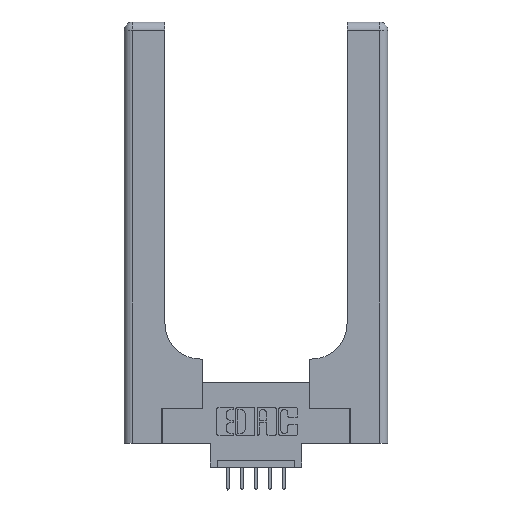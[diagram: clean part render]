
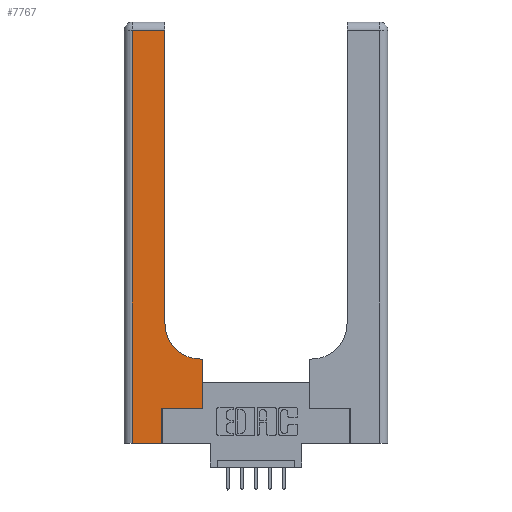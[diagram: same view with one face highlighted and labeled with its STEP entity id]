
A CAD part, top view. The second image highlights one B-rep face of the part: STEP entity #7767.
In plain terms, the highlighted planar face has unit normal (0, 0, 1).
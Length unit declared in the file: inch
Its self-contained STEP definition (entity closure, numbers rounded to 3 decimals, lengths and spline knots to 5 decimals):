
#170 = CARTESIAN_POINT ( 'NONE',  ( 0.5585, 0.6, 0.37 ) ) ;
#234 = DIRECTION ( 'NONE',  ( 0., 1., 0. ) ) ;
#961 = DIRECTION ( 'NONE',  ( 0., -1., 0. ) ) ;
#978 = DIRECTION ( 'NONE',  ( 0., 1., 0. ) ) ;
#1142 = LINE ( 'NONE', #6953, #4225 ) ;
#1166 = VECTOR ( 'NONE', #961, 39.37008 ) ;
#1433 = CIRCLE ( 'NONE', #10699, 0.25 ) ;
#1473 = LINE ( 'NONE', #1996, #12757 ) ;
#1967 = EDGE_CURVE ( 'NONE', #4353, #11476, #1142, .T. ) ;
#1996 = CARTESIAN_POINT ( 'NONE',  ( 0.269, 0.25, 0.37 ) ) ;
#2134 = ORIENTED_EDGE ( 'NONE', *, *, #12451, .T. ) ;
#2267 = PLANE ( 'NONE',  #4599 ) ;
#2344 = ORIENTED_EDGE ( 'NONE', *, *, #4306, .T. ) ;
#2591 = ORIENTED_EDGE ( 'NONE', *, *, #8455, .T. ) ;
#2785 = ORIENTED_EDGE ( 'NONE', *, *, #5712, .T. ) ;
#2977 = VERTEX_POINT ( 'NONE', #9577 ) ;
#3075 = CARTESIAN_POINT ( 'NONE',  ( 0.06, 3., 0.37 ) ) ;
#3300 = LINE ( 'NONE', #5132, #11838 ) ;
#3360 = CARTESIAN_POINT ( 'NONE',  ( 0., 3., 0.37 ) ) ;
#3619 = CARTESIAN_POINT ( 'NONE',  ( 0.2915, 2.94, 0.37 ) ) ;
#3809 = CARTESIAN_POINT ( 'NONE',  ( 0., 2.94, 0.37 ) ) ;
#3987 = EDGE_CURVE ( 'NONE', #8454, #4376, #9463, .T. ) ;
#4225 = VECTOR ( 'NONE', #6894, 39.37008 ) ;
#4274 = VERTEX_POINT ( 'NONE', #13783 ) ;
#4306 = EDGE_CURVE ( 'NONE', #11476, #5413, #4666, .T. ) ;
#4353 = VERTEX_POINT ( 'NONE', #14012 ) ;
#4376 = VERTEX_POINT ( 'NONE', #170 ) ;
#4588 = CARTESIAN_POINT ( 'NONE',  ( 0.2915, 0.6, 0.37 ) ) ;
#4599 = AXIS2_PLACEMENT_3D ( 'NONE', #3360, #6526, #10893 ) ;
#4666 = LINE ( 'NONE', #7544, #11666 ) ;
#4766 = EDGE_CURVE ( 'NONE', #4274, #4353, #7361, .T. ) ;
#5132 = CARTESIAN_POINT ( 'NONE',  ( 0.2915, 3., 0.37 ) ) ;
#5268 = LINE ( 'NONE', #3809, #12948 ) ;
#5413 = VERTEX_POINT ( 'NONE', #13988 ) ;
#5712 = EDGE_CURVE ( 'NONE', #11669, #4274, #5268, .T. ) ;
#5795 = DIRECTION ( 'NONE',  ( -1., 0., 0. ) ) ;
#6062 = VECTOR ( 'NONE', #5795, 39.37008 ) ;
#6109 = DIRECTION ( 'NONE',  ( -1., 0., 0. ) ) ;
#6526 = DIRECTION ( 'NONE',  ( 0., 0., -1. ) ) ;
#6568 = VECTOR ( 'NONE', #234, 39.37008 ) ;
#6671 = ORIENTED_EDGE ( 'NONE', *, *, #3987, .T. ) ;
#6894 = DIRECTION ( 'NONE',  ( 1., 0., 0. ) ) ;
#6953 = CARTESIAN_POINT ( 'NONE',  ( 0., 0., 0.37 ) ) ;
#7361 = LINE ( 'NONE', #3075, #1166 ) ;
#7544 = CARTESIAN_POINT ( 'NONE',  ( 0.269, 0., 0.37 ) ) ;
#7767 = ADVANCED_FACE ( 'NONE', ( #12578 ), #2267, .F. ) ;
#8225 = ORIENTED_EDGE ( 'NONE', *, *, #13757, .T. ) ;
#8313 = CARTESIAN_POINT ( 'NONE',  ( 0.5415, 0.6, 0.37 ) ) ;
#8454 = VERTEX_POINT ( 'NONE', #10112 ) ;
#8455 = EDGE_CURVE ( 'NONE', #4376, #13713, #10314, .T. ) ;
#8727 = ORIENTED_EDGE ( 'NONE', *, *, #1967, .T. ) ;
#8873 = CARTESIAN_POINT ( 'NONE',  ( 0.5585, 0.25, 0.37 ) ) ;
#8997 = EDGE_CURVE ( 'NONE', #2977, #11669, #3300, .T. ) ;
#9305 = DIRECTION ( 'NONE',  ( 0., 0., -1. ) ) ;
#9463 = LINE ( 'NONE', #8873, #6568 ) ;
#9577 = CARTESIAN_POINT ( 'NONE',  ( 0.2915, 0.85, 0.37 ) ) ;
#9580 = DIRECTION ( 'NONE',  ( 1., 0., 0. ) ) ;
#10112 = CARTESIAN_POINT ( 'NONE',  ( 0.5585, 0.25, 0.37 ) ) ;
#10314 = LINE ( 'NONE', #4588, #6062 ) ;
#10393 = DIRECTION ( 'NONE',  ( 1., 0., 0. ) ) ;
#10400 = ORIENTED_EDGE ( 'NONE', *, *, #8997, .T. ) ;
#10699 = AXIS2_PLACEMENT_3D ( 'NONE', #11489, #9305, #10393 ) ;
#10893 = DIRECTION ( 'NONE',  ( -1., 0., 0. ) ) ;
#10961 = CARTESIAN_POINT ( 'NONE',  ( 0.269, 0., 0.37 ) ) ;
#11476 = VERTEX_POINT ( 'NONE', #10961 ) ;
#11489 = CARTESIAN_POINT ( 'NONE',  ( 0.5415, 0.85, 0.37 ) ) ;
#11666 = VECTOR ( 'NONE', #978, 39.37008 ) ;
#11669 = VERTEX_POINT ( 'NONE', #3619 ) ;
#11816 = ORIENTED_EDGE ( 'NONE', *, *, #4766, .T. ) ;
#11838 = VECTOR ( 'NONE', #13723, 39.37008 ) ;
#12451 = EDGE_CURVE ( 'NONE', #5413, #8454, #1473, .T. ) ;
#12578 = FACE_OUTER_BOUND ( 'NONE', #14118, .T. ) ;
#12757 = VECTOR ( 'NONE', #9580, 39.37008 ) ;
#12948 = VECTOR ( 'NONE', #6109, 39.37008 ) ;
#13713 = VERTEX_POINT ( 'NONE', #8313 ) ;
#13723 = DIRECTION ( 'NONE',  ( 0., 1., 0. ) ) ;
#13757 = EDGE_CURVE ( 'NONE', #13713, #2977, #1433, .T. ) ;
#13783 = CARTESIAN_POINT ( 'NONE',  ( 0.06, 2.94, 0.37 ) ) ;
#13988 = CARTESIAN_POINT ( 'NONE',  ( 0.269, 0.25, 0.37 ) ) ;
#14012 = CARTESIAN_POINT ( 'NONE',  ( 0.06, 0., 0.37 ) ) ;
#14118 = EDGE_LOOP ( 'NONE', ( #10400, #2785, #11816, #8727, #2344, #2134, #6671, #2591, #8225 ) ) ;
